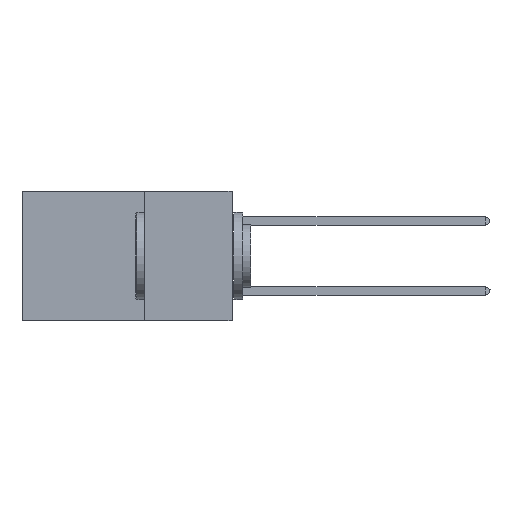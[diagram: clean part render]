
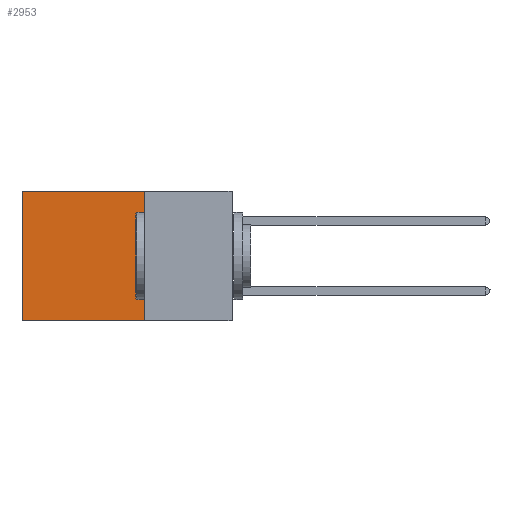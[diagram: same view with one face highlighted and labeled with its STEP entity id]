
A CAD part, left-side view. The second image highlights one B-rep face of the part: STEP entity #2953.
In plain terms, the highlighted planar face has unit normal (-1, 0, 0).
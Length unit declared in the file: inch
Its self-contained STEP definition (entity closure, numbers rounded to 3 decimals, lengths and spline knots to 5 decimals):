
#355 = VECTOR ( 'NONE', #7401, 39.37008 ) ;
#673 = DIRECTION ( 'NONE',  ( 0., 1., 0. ) ) ;
#832 = FACE_OUTER_BOUND ( 'NONE', #13135, .T. ) ;
#1181 = LINE ( 'NONE', #14742, #13391 ) ;
#1935 = DIRECTION ( 'NONE',  ( 1., 0., 0. ) ) ;
#2953 = ADVANCED_FACE ( 'NONE', ( #832 ), #3731, .F. ) ;
#3462 = CARTESIAN_POINT ( 'NONE',  ( 0.2875, 0.6, 0. ) ) ;
#3731 = PLANE ( 'NONE',  #4113 ) ;
#4113 = AXIS2_PLACEMENT_3D ( 'NONE', #13635, #1935, #17356 ) ;
#4794 = EDGE_CURVE ( 'NONE', #20686, #8091, #19900, .T. ) ;
#4993 = VERTEX_POINT ( 'NONE', #19303 ) ;
#5856 = EDGE_CURVE ( 'NONE', #8091, #4993, #18010, .T. ) ;
#7401 = DIRECTION ( 'NONE',  ( 0., 0., -1. ) ) ;
#8091 = VERTEX_POINT ( 'NONE', #16294 ) ;
#9293 = VECTOR ( 'NONE', #10985, 39.37008 ) ;
#9644 = CARTESIAN_POINT ( 'NONE',  ( 0.2875, 0.25, 0. ) ) ;
#10985 = DIRECTION ( 'NONE',  ( 0., 1., 0. ) ) ;
#13135 = EDGE_LOOP ( 'NONE', ( #14968, #24367, #24106, #16110 ) ) ;
#13391 = VECTOR ( 'NONE', #20322, 39.37008 ) ;
#13635 = CARTESIAN_POINT ( 'NONE',  ( 0.2875, 0.25, 0. ) ) ;
#14742 = CARTESIAN_POINT ( 'NONE',  ( 0.2875, 0.25, 0. ) ) ;
#14968 = ORIENTED_EDGE ( 'NONE', *, *, #5856, .T. ) ;
#16110 = ORIENTED_EDGE ( 'NONE', *, *, #4794, .T. ) ;
#16294 = CARTESIAN_POINT ( 'NONE',  ( 0.2875, 0.6, 0. ) ) ;
#16300 = VECTOR ( 'NONE', #673, 39.37008 ) ;
#17066 = EDGE_CURVE ( 'NONE', #19674, #4993, #21454, .T. ) ;
#17356 = DIRECTION ( 'NONE',  ( 0., 0., -1. ) ) ;
#18010 = LINE ( 'NONE', #3462, #355 ) ;
#19303 = CARTESIAN_POINT ( 'NONE',  ( 0.2875, 0.6, -0.37 ) ) ;
#19674 = VERTEX_POINT ( 'NONE', #24019 ) ;
#19900 = LINE ( 'NONE', #24643, #9293 ) ;
#20322 = DIRECTION ( 'NONE',  ( 0., 0., -1. ) ) ;
#20686 = VERTEX_POINT ( 'NONE', #9644 ) ;
#21454 = LINE ( 'NONE', #23965, #16300 ) ;
#22725 = EDGE_CURVE ( 'NONE', #20686, #19674, #1181, .T. ) ;
#23965 = CARTESIAN_POINT ( 'NONE',  ( 0.2875, 0.25, -0.37 ) ) ;
#24019 = CARTESIAN_POINT ( 'NONE',  ( 0.2875, 0.25, -0.37 ) ) ;
#24106 = ORIENTED_EDGE ( 'NONE', *, *, #22725, .F. ) ;
#24367 = ORIENTED_EDGE ( 'NONE', *, *, #17066, .F. ) ;
#24643 = CARTESIAN_POINT ( 'NONE',  ( 0.2875, 0.25, 0. ) ) ;
